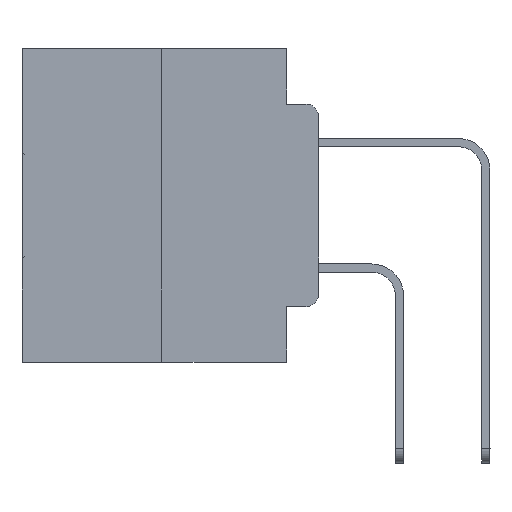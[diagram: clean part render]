
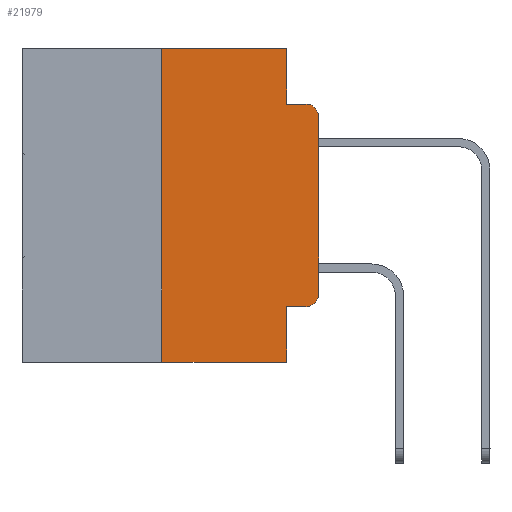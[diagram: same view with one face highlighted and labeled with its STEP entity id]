
A CAD part, left-side view. The second image highlights one B-rep face of the part: STEP entity #21979.
In plain terms, the highlighted planar face has unit normal (-1, 0, 0).
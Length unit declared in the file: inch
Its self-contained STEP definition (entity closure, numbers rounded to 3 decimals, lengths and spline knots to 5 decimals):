
#188 = EDGE_CURVE ( 'NONE', #24703, #16607, #20277, .T. ) ;
#1249 = LINE ( 'NONE', #14251, #26812 ) ;
#1369 = PLANE ( 'NONE',  #5792 ) ;
#1408 = CARTESIAN_POINT ( 'NONE',  ( 0., 0.051, 0. ) ) ;
#2077 = DIRECTION ( 'NONE',  ( 0., 0., -1. ) ) ;
#2198 = CARTESIAN_POINT ( 'NONE',  ( 0., 0.25, 0. ) ) ;
#2713 = CARTESIAN_POINT ( 'NONE',  ( 0., 0.051, 0. ) ) ;
#3237 = CARTESIAN_POINT ( 'NONE',  ( 0., 0.473, 0. ) ) ;
#4054 = AXIS2_PLACEMENT_3D ( 'NONE', #25754, #30640, #18007 ) ;
#4840 = EDGE_CURVE ( 'NONE', #21788, #25561, #14276, .T. ) ;
#5489 = CARTESIAN_POINT ( 'NONE',  ( 0., 0., -0.1085 ) ) ;
#5515 = VERTEX_POINT ( 'NONE', #27972 ) ;
#5782 = ORIENTED_EDGE ( 'NONE', *, *, #16082, .T. ) ;
#5792 = AXIS2_PLACEMENT_3D ( 'NONE', #11203, #28160, #6052 ) ;
#6052 = DIRECTION ( 'NONE',  ( 0., 0., -1. ) ) ;
#6936 = EDGE_CURVE ( 'NONE', #25561, #8043, #11698, .T. ) ;
#7051 = DIRECTION ( 'NONE',  ( 0., 0., 1. ) ) ;
#7846 = DIRECTION ( 'NONE',  ( 0., -1., 0. ) ) ;
#8043 = VERTEX_POINT ( 'NONE', #5489 ) ;
#8339 = CARTESIAN_POINT ( 'NONE',  ( 0., 0.051, -0.0885 ) ) ;
#8622 = AXIS2_PLACEMENT_3D ( 'NONE', #9359, #26617, #2077 ) ;
#8689 = ORIENTED_EDGE ( 'NONE', *, *, #28417, .F. ) ;
#9112 = ORIENTED_EDGE ( 'NONE', *, *, #26801, .F. ) ;
#9359 = CARTESIAN_POINT ( 'NONE',  ( 0., 0.02, -0.3915 ) ) ;
#9745 = VERTEX_POINT ( 'NONE', #2713 ) ;
#10322 = CARTESIAN_POINT ( 'NONE',  ( 0., 0.051, -0.4115 ) ) ;
#11058 = VECTOR ( 'NONE', #30305, 39.37008 ) ;
#11165 = VECTOR ( 'NONE', #7846, 39.37008 ) ;
#11203 = CARTESIAN_POINT ( 'NONE',  ( 0., 0.473, 0. ) ) ;
#11698 = LINE ( 'NONE', #21524, #26739 ) ;
#12714 = CARTESIAN_POINT ( 'NONE',  ( 0., 0.25, -0.5 ) ) ;
#12766 = DIRECTION ( 'NONE',  ( 0., -1., 0. ) ) ;
#13456 = EDGE_CURVE ( 'NONE', #5515, #9745, #23064, .T. ) ;
#13477 = DIRECTION ( 'NONE',  ( 0., 0., 1. ) ) ;
#13900 = ORIENTED_EDGE ( 'NONE', *, *, #13456, .F. ) ;
#14074 = CARTESIAN_POINT ( 'NONE',  ( 0., 0.051, -0.5 ) ) ;
#14251 = CARTESIAN_POINT ( 'NONE',  ( 0., 0.051, 0. ) ) ;
#14269 = EDGE_CURVE ( 'NONE', #26169, #21788, #20554, .T. ) ;
#14276 = CIRCLE ( 'NONE', #8622, 0.02 ) ;
#14931 = LINE ( 'NONE', #2198, #16003 ) ;
#15999 = VECTOR ( 'NONE', #17877, 39.37008 ) ;
#16003 = VECTOR ( 'NONE', #7051, 39.37008 ) ;
#16082 = EDGE_CURVE ( 'NONE', #8043, #16607, #28293, .T. ) ;
#16607 = VERTEX_POINT ( 'NONE', #30910 ) ;
#17222 = VERTEX_POINT ( 'NONE', #12714 ) ;
#17683 = EDGE_CURVE ( 'NONE', #17222, #5515, #14931, .T. ) ;
#17877 = DIRECTION ( 'NONE',  ( 0., 0., -1. ) ) ;
#18007 = DIRECTION ( 'NONE',  ( 0., 0., -1. ) ) ;
#18881 = CARTESIAN_POINT ( 'NONE',  ( 0., 0.051, -0.0885 ) ) ;
#18928 = EDGE_LOOP ( 'NONE', ( #27740, #5782, #26599, #9112, #13900, #23648, #31538, #8689, #26469, #30264 ) ) ;
#19238 = CARTESIAN_POINT ( 'NONE',  ( 0., 0., -0.3915 ) ) ;
#20243 = CARTESIAN_POINT ( 'NONE',  ( 0., 0.02, -0.4115 ) ) ;
#20277 = LINE ( 'NONE', #8339, #11058 ) ;
#20554 = LINE ( 'NONE', #29967, #11165 ) ;
#21524 = CARTESIAN_POINT ( 'NONE',  ( 0., 0., 0. ) ) ;
#21788 = VERTEX_POINT ( 'NONE', #20243 ) ;
#21979 = ADVANCED_FACE ( 'NONE', ( #23468 ), #1369, .F. ) ;
#22933 = CARTESIAN_POINT ( 'NONE',  ( 0., 0.473, -0.5 ) ) ;
#23064 = LINE ( 'NONE', #3237, #23484 ) ;
#23468 = FACE_OUTER_BOUND ( 'NONE', #18928, .T. ) ;
#23484 = VECTOR ( 'NONE', #30205, 39.37008 ) ;
#23648 = ORIENTED_EDGE ( 'NONE', *, *, #17683, .F. ) ;
#24505 = EDGE_CURVE ( 'NONE', #17222, #30731, #30376, .T. ) ;
#24703 = VERTEX_POINT ( 'NONE', #18881 ) ;
#25561 = VERTEX_POINT ( 'NONE', #19238 ) ;
#25612 = LINE ( 'NONE', #1408, #15999 ) ;
#25754 = CARTESIAN_POINT ( 'NONE',  ( 0., 0.02, -0.1085 ) ) ;
#26169 = VERTEX_POINT ( 'NONE', #10322 ) ;
#26469 = ORIENTED_EDGE ( 'NONE', *, *, #14269, .T. ) ;
#26599 = ORIENTED_EDGE ( 'NONE', *, *, #188, .F. ) ;
#26617 = DIRECTION ( 'NONE',  ( -1., 0., 0. ) ) ;
#26739 = VECTOR ( 'NONE', #13477, 39.37008 ) ;
#26801 = EDGE_CURVE ( 'NONE', #9745, #24703, #1249, .T. ) ;
#26812 = VECTOR ( 'NONE', #28348, 39.37008 ) ;
#27740 = ORIENTED_EDGE ( 'NONE', *, *, #6936, .T. ) ;
#27972 = CARTESIAN_POINT ( 'NONE',  ( 0., 0.25, 0. ) ) ;
#28160 = DIRECTION ( 'NONE',  ( 1., 0., 0. ) ) ;
#28293 = CIRCLE ( 'NONE', #4054, 0.02 ) ;
#28348 = DIRECTION ( 'NONE',  ( 0., 0., -1. ) ) ;
#28417 = EDGE_CURVE ( 'NONE', #26169, #30731, #25612, .T. ) ;
#29562 = VECTOR ( 'NONE', #12766, 39.37008 ) ;
#29967 = CARTESIAN_POINT ( 'NONE',  ( 0., 0.051, -0.4115 ) ) ;
#30205 = DIRECTION ( 'NONE',  ( 0., -1., 0. ) ) ;
#30264 = ORIENTED_EDGE ( 'NONE', *, *, #4840, .T. ) ;
#30305 = DIRECTION ( 'NONE',  ( 0., -1., 0. ) ) ;
#30376 = LINE ( 'NONE', #22933, #29562 ) ;
#30640 = DIRECTION ( 'NONE',  ( -1., 0., 0. ) ) ;
#30731 = VERTEX_POINT ( 'NONE', #14074 ) ;
#30910 = CARTESIAN_POINT ( 'NONE',  ( 0., 0.02, -0.0885 ) ) ;
#31538 = ORIENTED_EDGE ( 'NONE', *, *, #24505, .T. ) ;
